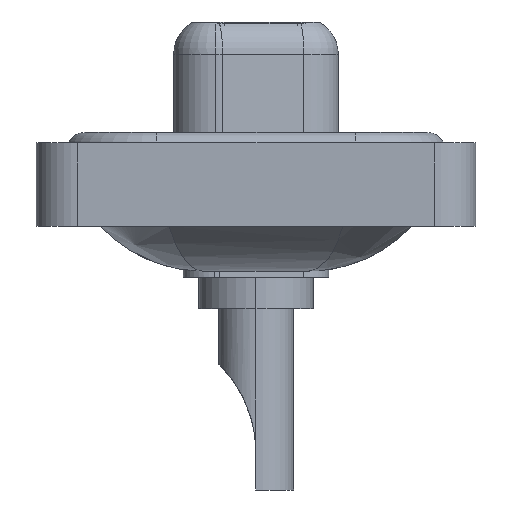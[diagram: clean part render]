
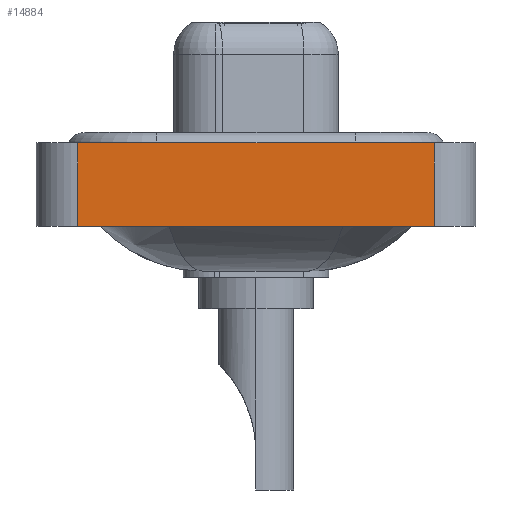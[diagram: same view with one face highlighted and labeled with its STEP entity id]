
A CAD part, left-side view. The second image highlights one B-rep face of the part: STEP entity #14884.
In plain terms, the highlighted planar face has unit normal (-1, 0, 0).
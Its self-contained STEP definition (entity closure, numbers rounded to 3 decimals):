
#636 = ORIENTED_EDGE ( 'NONE', *, *, #7418, .F. ) ;
#688 = AXIS2_PLACEMENT_3D ( 'NONE', #12073, #13579, #15093 ) ;
#721 = EDGE_CURVE ( 'NONE', #11294, #15763, #11094, .T. ) ;
#1870 = DIRECTION ( 'NONE',  ( 0., -1., 0. ) ) ;
#2880 = CARTESIAN_POINT ( 'NONE',  ( -7.3, 8.55, 0.4 ) ) ;
#3244 = ORIENTED_EDGE ( 'NONE', *, *, #6047, .F. ) ;
#3314 = LINE ( 'NONE', #11672, #15578 ) ;
#4270 = DIRECTION ( 'NONE',  ( 0., 0., 1. ) ) ;
#4527 = VECTOR ( 'NONE', #4270, 1000. ) ;
#4781 = DIRECTION ( 'NONE',  ( 0., -1., 0. ) ) ;
#4887 = LINE ( 'NONE', #14543, #5042 ) ;
#5042 = VECTOR ( 'NONE', #4781, 1000. ) ;
#5238 = EDGE_CURVE ( 'NONE', #13729, #11294, #3314, .T. ) ;
#6028 = CARTESIAN_POINT ( 'NONE',  ( -7.3, 8.55, -3.6 ) ) ;
#6047 = EDGE_CURVE ( 'NONE', #13584, #15763, #4887, .T. ) ;
#6110 = CARTESIAN_POINT ( 'NONE',  ( -7.3, -8.55, -3.6 ) ) ;
#6258 = CARTESIAN_POINT ( 'NONE',  ( -7.3, 8.55, -3.6 ) ) ;
#6789 = FACE_OUTER_BOUND ( 'NONE', #11963, .T. ) ;
#7418 = EDGE_CURVE ( 'NONE', #13729, #13584, #15632, .T. ) ;
#7810 = VECTOR ( 'NONE', #11536, 1000. ) ;
#8058 = PLANE ( 'NONE',  #688 ) ;
#10716 = ORIENTED_EDGE ( 'NONE', *, *, #5238, .T. ) ;
#11094 = LINE ( 'NONE', #16528, #4527 ) ;
#11294 = VERTEX_POINT ( 'NONE', #6110 ) ;
#11536 = DIRECTION ( 'NONE',  ( 0., 0., 1. ) ) ;
#11672 = CARTESIAN_POINT ( 'NONE',  ( -7.3, -8.55, -3.6 ) ) ;
#11963 = EDGE_LOOP ( 'NONE', ( #12977, #3244, #636, #10716 ) ) ;
#12073 = CARTESIAN_POINT ( 'NONE',  ( -7.3, -8.55, -3.6 ) ) ;
#12977 = ORIENTED_EDGE ( 'NONE', *, *, #721, .T. ) ;
#13579 = DIRECTION ( 'NONE',  ( -1., 0., 0. ) ) ;
#13584 = VERTEX_POINT ( 'NONE', #2880 ) ;
#13729 = VERTEX_POINT ( 'NONE', #6028 ) ;
#14543 = CARTESIAN_POINT ( 'NONE',  ( -7.3, -8.55, 0.4 ) ) ;
#14884 = ADVANCED_FACE ( 'NONE', ( #6789 ), #8058, .T. ) ;
#14984 = CARTESIAN_POINT ( 'NONE',  ( -7.3, -8.55, 0.4 ) ) ;
#15093 = DIRECTION ( 'NONE',  ( 0., 0., 1. ) ) ;
#15578 = VECTOR ( 'NONE', #1870, 1000. ) ;
#15632 = LINE ( 'NONE', #6258, #7810 ) ;
#15763 = VERTEX_POINT ( 'NONE', #14984 ) ;
#16528 = CARTESIAN_POINT ( 'NONE',  ( -7.3, -8.55, -3.6 ) ) ;
